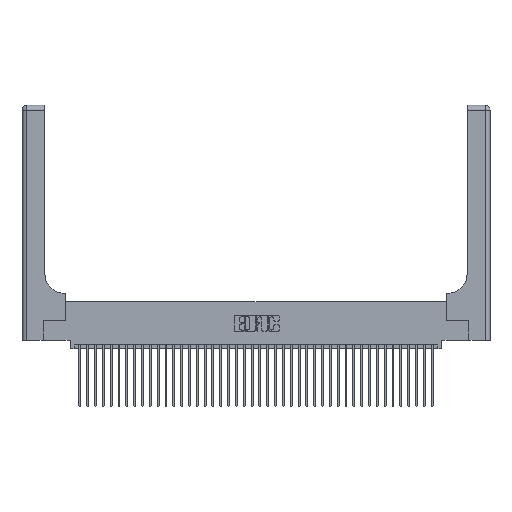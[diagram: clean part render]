
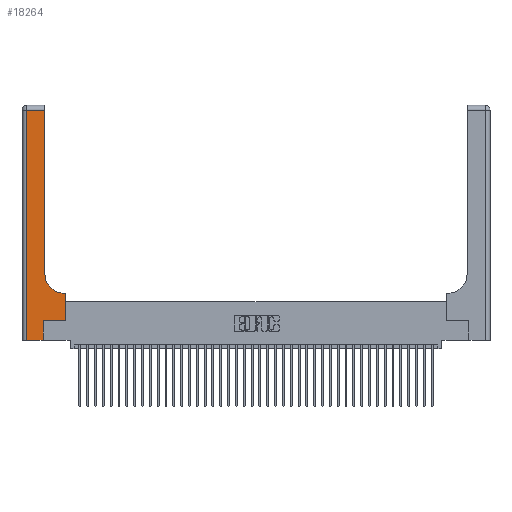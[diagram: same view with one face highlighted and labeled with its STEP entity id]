
A CAD part, top view. The second image highlights one B-rep face of the part: STEP entity #18264.
In plain terms, the highlighted planar face has unit normal (0, 0, 1).
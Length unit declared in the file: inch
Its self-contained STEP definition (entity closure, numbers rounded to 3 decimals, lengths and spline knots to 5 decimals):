
#305 = ORIENTED_EDGE ( 'NONE', *, *, #4385, .T. ) ;
#1360 = CARTESIAN_POINT ( 'NONE',  ( 0.269, 0.25, 0.37 ) ) ;
#2099 = DIRECTION ( 'NONE',  ( 1., 0., 0. ) ) ;
#2157 = EDGE_LOOP ( 'NONE', ( #29660, #39424, #11638, #10264, #305, #17228, #20233, #27117, #11289 ) ) ;
#2454 = CARTESIAN_POINT ( 'NONE',  ( 0., 0., 0.37 ) ) ;
#2870 = CARTESIAN_POINT ( 'NONE',  ( 0.269, 0., 0.37 ) ) ;
#3420 = LINE ( 'NONE', #35261, #11886 ) ;
#3558 = CARTESIAN_POINT ( 'NONE',  ( 0.5585, 0.25, 0.37 ) ) ;
#3833 = AXIS2_PLACEMENT_3D ( 'NONE', #17445, #26944, #7984 ) ;
#3917 = CARTESIAN_POINT ( 'NONE',  ( 0.2915, 2.94, 0.37 ) ) ;
#4385 = EDGE_CURVE ( 'NONE', #32447, #20991, #35091, .T. ) ;
#4785 = PLANE ( 'NONE',  #3833 ) ;
#6454 = CARTESIAN_POINT ( 'NONE',  ( 0.06, 3., 0.37 ) ) ;
#7984 = DIRECTION ( 'NONE',  ( -1., 0., 0. ) ) ;
#10264 = ORIENTED_EDGE ( 'NONE', *, *, #21154, .T. ) ;
#10882 = VERTEX_POINT ( 'NONE', #3917 ) ;
#11289 = ORIENTED_EDGE ( 'NONE', *, *, #13259, .T. ) ;
#11331 = FACE_OUTER_BOUND ( 'NONE', #2157, .T. ) ;
#11478 = CARTESIAN_POINT ( 'NONE',  ( 0.5585, 0.6, 0.37 ) ) ;
#11638 = ORIENTED_EDGE ( 'NONE', *, *, #28666, .T. ) ;
#11716 = LINE ( 'NONE', #2454, #35860 ) ;
#11886 = VECTOR ( 'NONE', #19635, 39.37008 ) ;
#12584 = VERTEX_POINT ( 'NONE', #11478 ) ;
#12854 = EDGE_CURVE ( 'NONE', #12584, #37627, #37132, .T. ) ;
#13259 = EDGE_CURVE ( 'NONE', #37627, #15412, #23371, .T. ) ;
#15412 = VERTEX_POINT ( 'NONE', #40638 ) ;
#15752 = DIRECTION ( 'NONE',  ( 0., 1., 0. ) ) ;
#15788 = VERTEX_POINT ( 'NONE', #23600 ) ;
#16351 = LINE ( 'NONE', #17917, #31175 ) ;
#17228 = ORIENTED_EDGE ( 'NONE', *, *, #17677, .T. ) ;
#17382 = CARTESIAN_POINT ( 'NONE',  ( 0.5585, 0.25, 0.37 ) ) ;
#17445 = CARTESIAN_POINT ( 'NONE',  ( 0., 3., 0.37 ) ) ;
#17677 = EDGE_CURVE ( 'NONE', #20991, #32602, #16351, .T. ) ;
#17917 = CARTESIAN_POINT ( 'NONE',  ( 0.269, 0.25, 0.37 ) ) ;
#18264 = ADVANCED_FACE ( 'NONE', ( #11331 ), #4785, .F. ) ;
#18651 = VECTOR ( 'NONE', #15752, 39.37008 ) ;
#19635 = DIRECTION ( 'NONE',  ( -1., 0., 0. ) ) ;
#20233 = ORIENTED_EDGE ( 'NONE', *, *, #30623, .T. ) ;
#20580 = DIRECTION ( 'NONE',  ( 0., 1., 0. ) ) ;
#20884 = VERTEX_POINT ( 'NONE', #23157 ) ;
#20991 = VERTEX_POINT ( 'NONE', #1360 ) ;
#21137 = DIRECTION ( 'NONE',  ( 0., 0., -1. ) ) ;
#21154 = EDGE_CURVE ( 'NONE', #20884, #32447, #11716, .T. ) ;
#21488 = DIRECTION ( 'NONE',  ( 1., 0., 0. ) ) ;
#21887 = EDGE_CURVE ( 'NONE', #15412, #10882, #26011, .T. ) ;
#22399 = DIRECTION ( 'NONE',  ( -1., 0., 0. ) ) ;
#23157 = CARTESIAN_POINT ( 'NONE',  ( 0.06, 0., 0.37 ) ) ;
#23371 = CIRCLE ( 'NONE', #38120, 0.25 ) ;
#23600 = CARTESIAN_POINT ( 'NONE',  ( 0.06, 2.94, 0.37 ) ) ;
#24560 = CARTESIAN_POINT ( 'NONE',  ( 0.5415, 0.6, 0.37 ) ) ;
#24833 = DIRECTION ( 'NONE',  ( 0., -1., 0. ) ) ;
#26011 = LINE ( 'NONE', #37740, #18651 ) ;
#26944 = DIRECTION ( 'NONE',  ( 0., 0., -1. ) ) ;
#27117 = ORIENTED_EDGE ( 'NONE', *, *, #12854, .T. ) ;
#28637 = CARTESIAN_POINT ( 'NONE',  ( 0.2915, 0.6, 0.37 ) ) ;
#28666 = EDGE_CURVE ( 'NONE', #15788, #20884, #29101, .T. ) ;
#28869 = VECTOR ( 'NONE', #22399, 39.37008 ) ;
#29101 = LINE ( 'NONE', #6454, #35434 ) ;
#29660 = ORIENTED_EDGE ( 'NONE', *, *, #21887, .T. ) ;
#29942 = CARTESIAN_POINT ( 'NONE',  ( 0.269, 0., 0.37 ) ) ;
#30623 = EDGE_CURVE ( 'NONE', #32602, #12584, #33316, .T. ) ;
#31175 = VECTOR ( 'NONE', #39851, 39.37008 ) ;
#32447 = VERTEX_POINT ( 'NONE', #2870 ) ;
#32602 = VERTEX_POINT ( 'NONE', #3558 ) ;
#33316 = LINE ( 'NONE', #17382, #40652 ) ;
#34119 = VECTOR ( 'NONE', #39079, 39.37008 ) ;
#35091 = LINE ( 'NONE', #29942, #34119 ) ;
#35261 = CARTESIAN_POINT ( 'NONE',  ( 0., 2.94, 0.37 ) ) ;
#35434 = VECTOR ( 'NONE', #24833, 39.37008 ) ;
#35860 = VECTOR ( 'NONE', #21488, 39.37008 ) ;
#37132 = LINE ( 'NONE', #28637, #28869 ) ;
#37627 = VERTEX_POINT ( 'NONE', #24560 ) ;
#37740 = CARTESIAN_POINT ( 'NONE',  ( 0.2915, 3., 0.37 ) ) ;
#38120 = AXIS2_PLACEMENT_3D ( 'NONE', #39916, #21137, #2099 ) ;
#39079 = DIRECTION ( 'NONE',  ( 0., 1., 0. ) ) ;
#39424 = ORIENTED_EDGE ( 'NONE', *, *, #39651, .T. ) ;
#39651 = EDGE_CURVE ( 'NONE', #10882, #15788, #3420, .T. ) ;
#39851 = DIRECTION ( 'NONE',  ( 1., 0., 0. ) ) ;
#39916 = CARTESIAN_POINT ( 'NONE',  ( 0.5415, 0.85, 0.37 ) ) ;
#40638 = CARTESIAN_POINT ( 'NONE',  ( 0.2915, 0.85, 0.37 ) ) ;
#40652 = VECTOR ( 'NONE', #20580, 39.37008 ) ;
